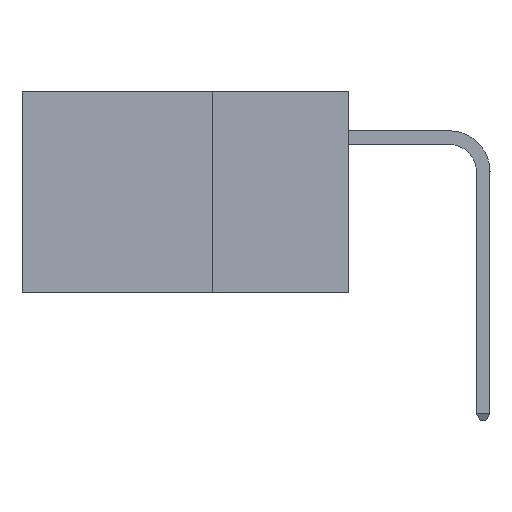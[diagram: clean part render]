
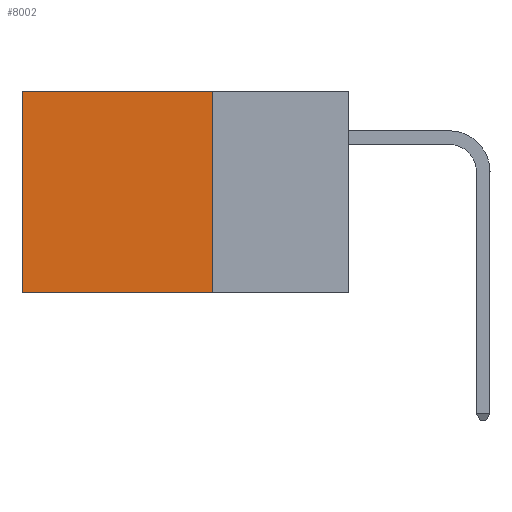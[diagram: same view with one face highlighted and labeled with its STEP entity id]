
A CAD part, left-side view. The second image highlights one B-rep face of the part: STEP entity #8002.
In plain terms, the highlighted planar face has unit normal (-1, 0, 0).
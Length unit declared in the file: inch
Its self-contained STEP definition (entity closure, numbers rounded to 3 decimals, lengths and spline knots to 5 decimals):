
#11 = CARTESIAN_POINT ( 'NONE',  ( 0.2875, 0.6, 0. ) ) ;
#1317 = DIRECTION ( 'NONE',  ( 0., 0., -1. ) ) ;
#1942 = VERTEX_POINT ( 'NONE', #4513 ) ;
#2372 = VERTEX_POINT ( 'NONE', #10532 ) ;
#2493 = CARTESIAN_POINT ( 'NONE',  ( 0.2875, 0.25, -0.37 ) ) ;
#2539 = VECTOR ( 'NONE', #13846, 39.37008 ) ;
#2836 = VECTOR ( 'NONE', #14242, 39.37008 ) ;
#3403 = CARTESIAN_POINT ( 'NONE',  ( 0.2875, 0.25, 0. ) ) ;
#4051 = PLANE ( 'NONE',  #7606 ) ;
#4133 = ORIENTED_EDGE ( 'NONE', *, *, #6901, .T. ) ;
#4428 = DIRECTION ( 'NONE',  ( 0., 1., 0. ) ) ;
#4513 = CARTESIAN_POINT ( 'NONE',  ( 0.2875, 0.6, 0. ) ) ;
#4717 = ORIENTED_EDGE ( 'NONE', *, *, #7946, .T. ) ;
#5641 = VECTOR ( 'NONE', #4428, 39.37008 ) ;
#5813 = VECTOR ( 'NONE', #1317, 39.37008 ) ;
#6234 = LINE ( 'NONE', #11, #5813 ) ;
#6375 = LINE ( 'NONE', #2493, #2836 ) ;
#6401 = EDGE_CURVE ( 'NONE', #7411, #2372, #16333, .T. ) ;
#6720 = DIRECTION ( 'NONE',  ( 1., 0., 0. ) ) ;
#6901 = EDGE_CURVE ( 'NONE', #7411, #1942, #9552, .T. ) ;
#7411 = VERTEX_POINT ( 'NONE', #11960 ) ;
#7606 = AXIS2_PLACEMENT_3D ( 'NONE', #11886, #6720, #15712 ) ;
#7946 = EDGE_CURVE ( 'NONE', #1942, #9568, #6234, .T. ) ;
#8002 = ADVANCED_FACE ( 'NONE', ( #15300 ), #4051, .F. ) ;
#9464 = EDGE_CURVE ( 'NONE', #2372, #9568, #6375, .T. ) ;
#9552 = LINE ( 'NONE', #10993, #5641 ) ;
#9568 = VERTEX_POINT ( 'NONE', #14398 ) ;
#10532 = CARTESIAN_POINT ( 'NONE',  ( 0.2875, 0.25, -0.37 ) ) ;
#10900 = EDGE_LOOP ( 'NONE', ( #4717, #13562, #12854, #4133 ) ) ;
#10993 = CARTESIAN_POINT ( 'NONE',  ( 0.2875, 0.25, 0. ) ) ;
#11886 = CARTESIAN_POINT ( 'NONE',  ( 0.2875, 0.25, 0. ) ) ;
#11960 = CARTESIAN_POINT ( 'NONE',  ( 0.2875, 0.25, 0. ) ) ;
#12854 = ORIENTED_EDGE ( 'NONE', *, *, #6401, .F. ) ;
#13562 = ORIENTED_EDGE ( 'NONE', *, *, #9464, .F. ) ;
#13846 = DIRECTION ( 'NONE',  ( 0., 0., -1. ) ) ;
#14242 = DIRECTION ( 'NONE',  ( 0., 1., 0. ) ) ;
#14398 = CARTESIAN_POINT ( 'NONE',  ( 0.2875, 0.6, -0.37 ) ) ;
#15300 = FACE_OUTER_BOUND ( 'NONE', #10900, .T. ) ;
#15712 = DIRECTION ( 'NONE',  ( 0., 0., -1. ) ) ;
#16333 = LINE ( 'NONE', #3403, #2539 ) ;
